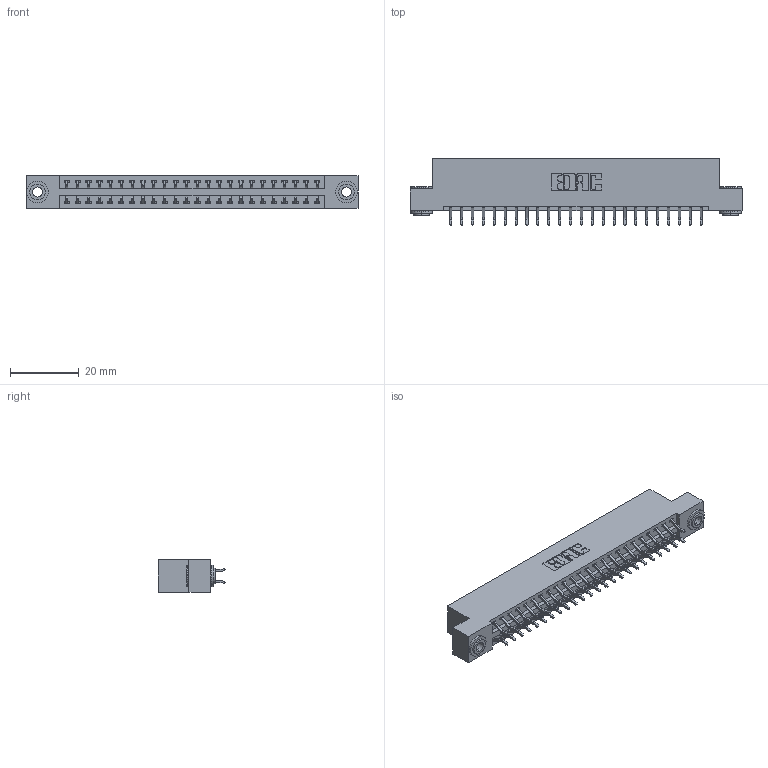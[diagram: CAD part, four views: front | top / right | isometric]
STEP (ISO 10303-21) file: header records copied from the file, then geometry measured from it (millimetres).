
FILE_DESCRIPTION (( 'STEP AP203' ), '1' );
FILE_NAME ('396-048-556-203.STEP', '2019-10-30T12:42:36', ( '' ), ( '' ), 'SwSTEP 2.0', 'SolidWorks 2016', '' );
FILE_SCHEMA (( 'CONFIG_CONTROL_DESIGN' ));
Length unit declared in the file: inch
Products named in the file (4): 346 Part_Flush Mounting Lugs - 0.156 Dia-TH; 396-048-556-203; 345-292-001_556 Tail; 345-250-002_345-250-002-102
Assembly tree (51 placements, depth 2):
  396-048-556-203
    346 Part_Flush Mounting Lugs - 0.156 Dia-TH
    345-292-001_556 Tail  x48
    345-250-002_345-250-002-102  x2
Bounding box: 96.77 x 19.57 x 9.4 mm (x, y, z)
Volume: 9314.4 mm3; surface area: 12689.9 mm2
Topology: 51 solids, 51 shells, 2944 faces, 8709 edges, 5738 vertices
Faces by surface type: plane 1958, cylinder 978, cone 8
Entity records: 18956 total; most frequent: CARTESIAN_POINT 3139, ORIENTED_EDGE 3054, DIRECTION 2837, EDGE_CURVE 1527, LINE 1267, VECTOR 1267, VERTEX_POINT 1014, AXIS2_PLACEMENT_3D 785
